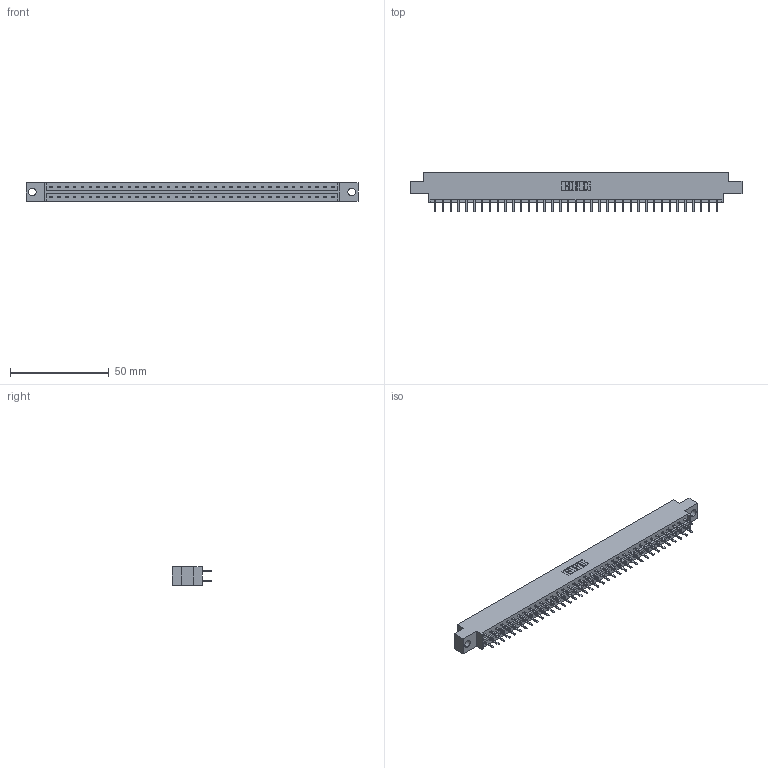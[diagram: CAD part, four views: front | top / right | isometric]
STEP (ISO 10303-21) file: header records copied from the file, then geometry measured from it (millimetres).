
FILE_DESCRIPTION (( 'STEP AP203' ), '1' );
FILE_NAME ('333-074-520-804.STEP', '2018-08-04T21:33:08', ( '' ), ( '' ), 'SwSTEP 2.0', 'SolidWorks 2016', '' );
FILE_SCHEMA (( 'CONFIG_CONTROL_DESIGN' ));
Length unit declared in the file: inch
Products named in the file (3): 333 Part_Offset - .156 Dia - TH; 345-292-001_345-293-120; 333-074-520-804
Assembly tree (75 placements, depth 2):
  333-074-520-804
    333 Part_Offset - .156 Dia - TH
    345-292-001_345-293-120  x74
Bounding box: 168.15 x 20.02 x 9.4 mm (x, y, z)
Volume: 16772 mm3; surface area: 19709.1 mm2
Topology: 75 solids, 75 shells, 4262 faces, 12385 edges, 8058 vertices
Faces by surface type: plane 2886, cylinder 1376
Entity records: 24699 total; most frequent: CARTESIAN_POINT 4114, ORIENTED_EDGE 4038, DIRECTION 3511, EDGE_CURVE 2019, LINE 1887, VECTOR 1887, VERTEX_POINT 1342, AXIS2_PLACEMENT_3D 812
